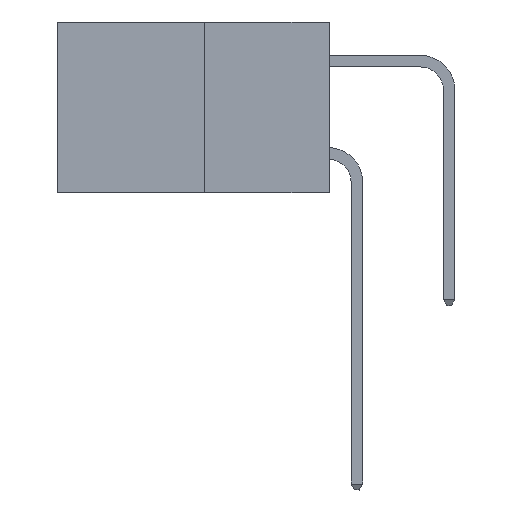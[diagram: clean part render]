
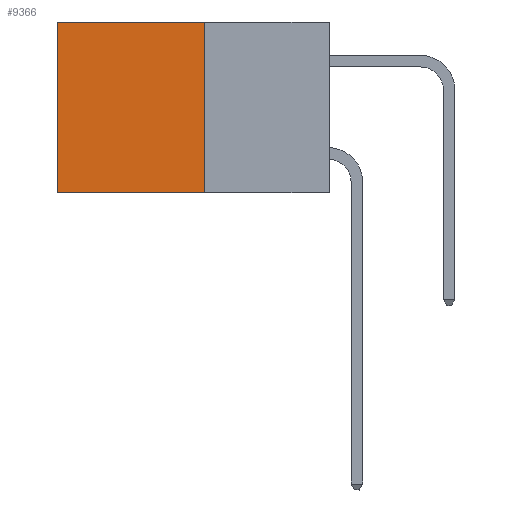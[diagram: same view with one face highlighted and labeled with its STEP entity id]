
A CAD part, left-side view. The second image highlights one B-rep face of the part: STEP entity #9366.
In plain terms, the highlighted planar face has unit normal (-1, 0, 0).
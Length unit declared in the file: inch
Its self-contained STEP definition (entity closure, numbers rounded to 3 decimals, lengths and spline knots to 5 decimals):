
#562 = LINE ( 'NONE', #9031, #10991 ) ;
#835 = VERTEX_POINT ( 'NONE', #10903 ) ;
#1865 = EDGE_LOOP ( 'NONE', ( #23728, #24463, #2126, #21458 ) ) ;
#1991 = LINE ( 'NONE', #11003, #13002 ) ;
#2126 = ORIENTED_EDGE ( 'NONE', *, *, #25201, .F. ) ;
#2263 = DIRECTION ( 'NONE',  ( 0., 1., 0. ) ) ;
#2540 = DIRECTION ( 'NONE',  ( 1., 0., 0. ) ) ;
#2692 = CARTESIAN_POINT ( 'NONE',  ( 0.277, 0.27, -0.37 ) ) ;
#3159 = VECTOR ( 'NONE', #22403, 39.37008 ) ;
#3602 = EDGE_CURVE ( 'NONE', #14929, #14289, #14196, .T. ) ;
#4717 = DIRECTION ( 'NONE',  ( 0., 0., -1. ) ) ;
#7021 = CARTESIAN_POINT ( 'NONE',  ( 0.277, 0.59, 0. ) ) ;
#7367 = EDGE_CURVE ( 'NONE', #11522, #835, #17228, .T. ) ;
#8310 = FACE_OUTER_BOUND ( 'NONE', #1865, .T. ) ;
#8697 = PLANE ( 'NONE',  #22380 ) ;
#9031 = CARTESIAN_POINT ( 'NONE',  ( 0.277, 0.59, -0.37 ) ) ;
#9366 = ADVANCED_FACE ( 'NONE', ( #8310 ), #8697, .F. ) ;
#10532 = CARTESIAN_POINT ( 'NONE',  ( 0.277, 0.27, -0.37 ) ) ;
#10635 = CARTESIAN_POINT ( 'NONE',  ( 0.277, 0.27, 0. ) ) ;
#10903 = CARTESIAN_POINT ( 'NONE',  ( 0.277, 0.59, -0.37 ) ) ;
#10991 = VECTOR ( 'NONE', #25536, 39.37008 ) ;
#11003 = CARTESIAN_POINT ( 'NONE',  ( 0.277, 0.27, -0.37 ) ) ;
#11522 = VERTEX_POINT ( 'NONE', #2692 ) ;
#11761 = VECTOR ( 'NONE', #2263, 39.37008 ) ;
#13002 = VECTOR ( 'NONE', #4717, 39.37008 ) ;
#13557 = EDGE_CURVE ( 'NONE', #14289, #835, #562, .T. ) ;
#14196 = LINE ( 'NONE', #20517, #3159 ) ;
#14289 = VERTEX_POINT ( 'NONE', #7021 ) ;
#14929 = VERTEX_POINT ( 'NONE', #10635 ) ;
#14944 = CARTESIAN_POINT ( 'NONE',  ( 0.277, 0.27, -0.37 ) ) ;
#16996 = DIRECTION ( 'NONE',  ( 0., 0., -1. ) ) ;
#17228 = LINE ( 'NONE', #10532, #11761 ) ;
#20517 = CARTESIAN_POINT ( 'NONE',  ( 0.277, 0.27, 0. ) ) ;
#21458 = ORIENTED_EDGE ( 'NONE', *, *, #3602, .T. ) ;
#22380 = AXIS2_PLACEMENT_3D ( 'NONE', #14944, #2540, #16996 ) ;
#22403 = DIRECTION ( 'NONE',  ( 0., 1., 0. ) ) ;
#23728 = ORIENTED_EDGE ( 'NONE', *, *, #13557, .T. ) ;
#24463 = ORIENTED_EDGE ( 'NONE', *, *, #7367, .F. ) ;
#25201 = EDGE_CURVE ( 'NONE', #14929, #11522, #1991, .T. ) ;
#25536 = DIRECTION ( 'NONE',  ( 0., 0., -1. ) ) ;
